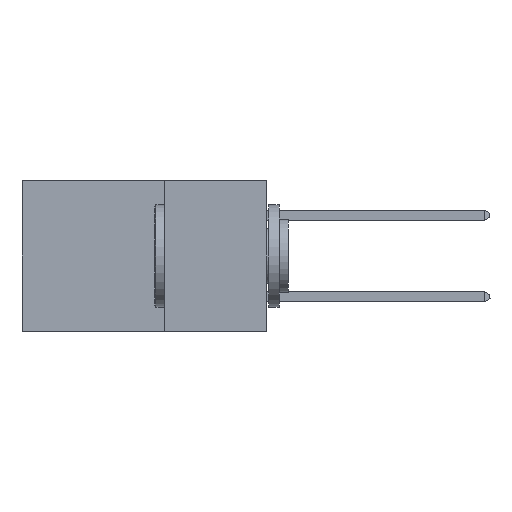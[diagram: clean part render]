
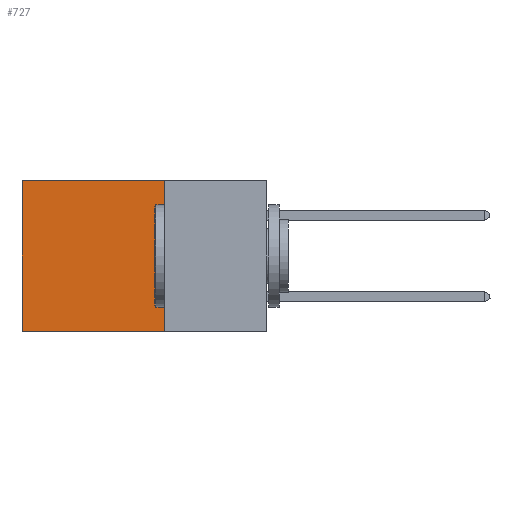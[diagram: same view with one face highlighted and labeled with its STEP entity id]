
A CAD part, left-side view. The second image highlights one B-rep face of the part: STEP entity #727.
In plain terms, the highlighted planar face has unit normal (-1, 0, 0).
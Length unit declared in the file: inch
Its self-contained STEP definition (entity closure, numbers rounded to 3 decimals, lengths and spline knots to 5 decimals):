
#550 = CARTESIAN_POINT ( 'NONE',  ( 0.2875, 0.25, 0. ) ) ;
#727 = ADVANCED_FACE ( 'NONE', ( #8380 ), #10928, .F. ) ;
#884 = CARTESIAN_POINT ( 'NONE',  ( 0.2875, 0.25, 0. ) ) ;
#1524 = VERTEX_POINT ( 'NONE', #9335 ) ;
#2324 = ORIENTED_EDGE ( 'NONE', *, *, #24813, .F. ) ;
#3443 = EDGE_LOOP ( 'NONE', ( #16895, #2324, #31476, #7534 ) ) ;
#5356 = DIRECTION ( 'NONE',  ( 0., 1., 0. ) ) ;
#5664 = CARTESIAN_POINT ( 'NONE',  ( 0.2875, 0.25, -0.37 ) ) ;
#6084 = VECTOR ( 'NONE', #29903, 39.37008 ) ;
#7189 = VECTOR ( 'NONE', #5356, 39.37008 ) ;
#7534 = ORIENTED_EDGE ( 'NONE', *, *, #19260, .T. ) ;
#8380 = FACE_OUTER_BOUND ( 'NONE', #3443, .T. ) ;
#8809 = CARTESIAN_POINT ( 'NONE',  ( 0.2875, 0.6, 0. ) ) ;
#9333 = LINE ( 'NONE', #21559, #23910 ) ;
#9335 = CARTESIAN_POINT ( 'NONE',  ( 0.2875, 0.6, -0.37 ) ) ;
#9824 = LINE ( 'NONE', #15676, #27021 ) ;
#10095 = CARTESIAN_POINT ( 'NONE',  ( 0.2875, 0.25, 0. ) ) ;
#10673 = DIRECTION ( 'NONE',  ( 0., 0., -1. ) ) ;
#10928 = PLANE ( 'NONE',  #17614 ) ;
#12581 = LINE ( 'NONE', #27337, #6084 ) ;
#14375 = DIRECTION ( 'NONE',  ( 0., 1., 0. ) ) ;
#15065 = EDGE_CURVE ( 'NONE', #21275, #1524, #9824, .T. ) ;
#15507 = VERTEX_POINT ( 'NONE', #10095 ) ;
#15676 = CARTESIAN_POINT ( 'NONE',  ( 0.2875, 0.6, 0. ) ) ;
#16895 = ORIENTED_EDGE ( 'NONE', *, *, #15065, .T. ) ;
#17476 = EDGE_CURVE ( 'NONE', #15507, #22743, #12581, .T. ) ;
#17614 = AXIS2_PLACEMENT_3D ( 'NONE', #884, #17995, #20449 ) ;
#17892 = LINE ( 'NONE', #550, #7189 ) ;
#17995 = DIRECTION ( 'NONE',  ( 1., 0., 0. ) ) ;
#19260 = EDGE_CURVE ( 'NONE', #15507, #21275, #17892, .T. ) ;
#20449 = DIRECTION ( 'NONE',  ( 0., 0., -1. ) ) ;
#21275 = VERTEX_POINT ( 'NONE', #8809 ) ;
#21559 = CARTESIAN_POINT ( 'NONE',  ( 0.2875, 0.25, -0.37 ) ) ;
#22743 = VERTEX_POINT ( 'NONE', #5664 ) ;
#23910 = VECTOR ( 'NONE', #14375, 39.37008 ) ;
#24813 = EDGE_CURVE ( 'NONE', #22743, #1524, #9333, .T. ) ;
#27021 = VECTOR ( 'NONE', #10673, 39.37008 ) ;
#27337 = CARTESIAN_POINT ( 'NONE',  ( 0.2875, 0.25, 0. ) ) ;
#29903 = DIRECTION ( 'NONE',  ( 0., 0., -1. ) ) ;
#31476 = ORIENTED_EDGE ( 'NONE', *, *, #17476, .F. ) ;
